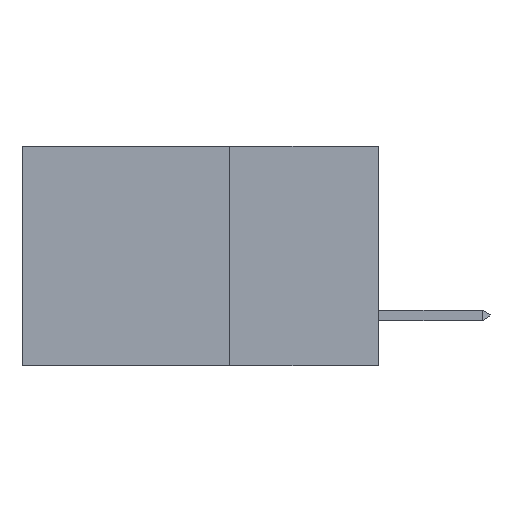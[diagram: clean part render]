
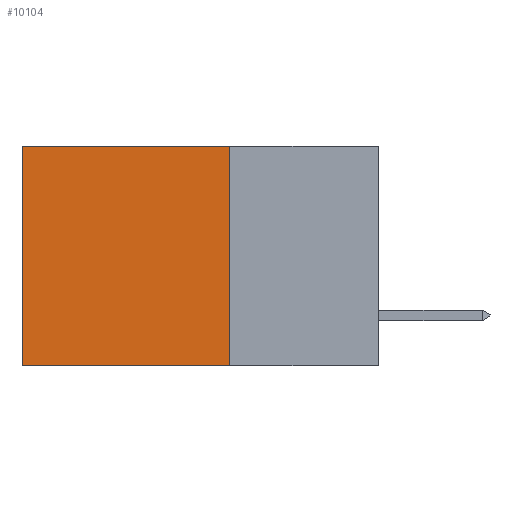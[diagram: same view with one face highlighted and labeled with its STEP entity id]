
A CAD part, left-side view. The second image highlights one B-rep face of the part: STEP entity #10104.
In plain terms, the highlighted planar face has unit normal (-1, 0, 0).
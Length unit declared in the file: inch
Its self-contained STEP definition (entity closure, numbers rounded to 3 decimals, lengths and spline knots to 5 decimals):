
#24 = DIRECTION ( 'NONE',  ( 0., 1., 0. ) ) ;
#378 = FACE_OUTER_BOUND ( 'NONE', #3338, .T. ) ;
#862 = VERTEX_POINT ( 'NONE', #11087 ) ;
#1357 = EDGE_CURVE ( 'NONE', #862, #10709, #7088, .T. ) ;
#1583 = DIRECTION ( 'NONE',  ( 0., 0., -1. ) ) ;
#2480 = DIRECTION ( 'NONE',  ( 0., 1., 0. ) ) ;
#2577 = ORIENTED_EDGE ( 'NONE', *, *, #1357, .F. ) ;
#2610 = CARTESIAN_POINT ( 'NONE',  ( 0.2615, 0.6, 0. ) ) ;
#3338 = EDGE_LOOP ( 'NONE', ( #4417, #2577, #7806, #8520 ) ) ;
#3480 = LINE ( 'NONE', #12563, #11330 ) ;
#3759 = PLANE ( 'NONE',  #12146 ) ;
#4417 = ORIENTED_EDGE ( 'NONE', *, *, #11770, .T. ) ;
#4906 = VECTOR ( 'NONE', #2480, 39.37008 ) ;
#5310 = EDGE_CURVE ( 'NONE', #9805, #862, #12485, .T. ) ;
#6620 = CARTESIAN_POINT ( 'NONE',  ( 0.2615, 0.6, -0.37 ) ) ;
#7083 = VECTOR ( 'NONE', #24, 39.37008 ) ;
#7088 = LINE ( 'NONE', #11121, #4906 ) ;
#7506 = DIRECTION ( 'NONE',  ( 1., 0., 0. ) ) ;
#7806 = ORIENTED_EDGE ( 'NONE', *, *, #5310, .F. ) ;
#8520 = ORIENTED_EDGE ( 'NONE', *, *, #10290, .T. ) ;
#8905 = DIRECTION ( 'NONE',  ( 0., 0., -1. ) ) ;
#9805 = VERTEX_POINT ( 'NONE', #9843 ) ;
#9843 = CARTESIAN_POINT ( 'NONE',  ( 0.2615, 0.25, 0. ) ) ;
#10104 = ADVANCED_FACE ( 'NONE', ( #378 ), #3759, .F. ) ;
#10290 = EDGE_CURVE ( 'NONE', #9805, #10656, #11989, .T. ) ;
#10583 = CARTESIAN_POINT ( 'NONE',  ( 0.2615, 0.25, -0.37 ) ) ;
#10656 = VERTEX_POINT ( 'NONE', #2610 ) ;
#10709 = VERTEX_POINT ( 'NONE', #6620 ) ;
#11053 = CARTESIAN_POINT ( 'NONE',  ( 0.2615, 0.25, 0. ) ) ;
#11087 = CARTESIAN_POINT ( 'NONE',  ( 0.2615, 0.25, -0.37 ) ) ;
#11121 = CARTESIAN_POINT ( 'NONE',  ( 0.2615, 0.25, -0.37 ) ) ;
#11330 = VECTOR ( 'NONE', #12690, 39.37008 ) ;
#11534 = CARTESIAN_POINT ( 'NONE',  ( 0.2615, 0.25, -0.37 ) ) ;
#11644 = VECTOR ( 'NONE', #1583, 39.37008 ) ;
#11770 = EDGE_CURVE ( 'NONE', #10656, #10709, #3480, .T. ) ;
#11989 = LINE ( 'NONE', #11053, #7083 ) ;
#12146 = AXIS2_PLACEMENT_3D ( 'NONE', #11534, #7506, #8905 ) ;
#12485 = LINE ( 'NONE', #10583, #11644 ) ;
#12563 = CARTESIAN_POINT ( 'NONE',  ( 0.2615, 0.6, -0.37 ) ) ;
#12690 = DIRECTION ( 'NONE',  ( 0., 0., -1. ) ) ;
